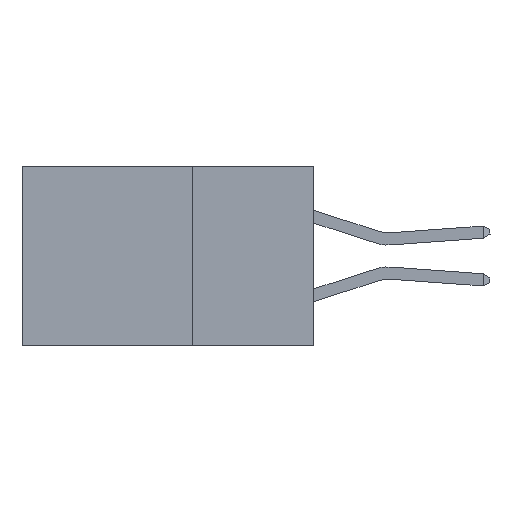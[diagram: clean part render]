
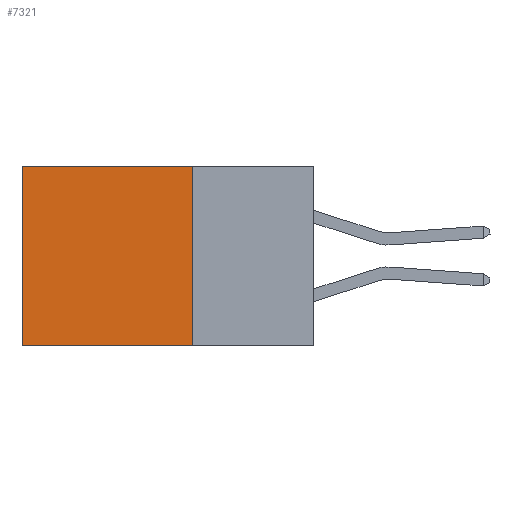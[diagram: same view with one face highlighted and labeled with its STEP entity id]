
A CAD part, left-side view. The second image highlights one B-rep face of the part: STEP entity #7321.
In plain terms, the highlighted planar face has unit normal (-1, 0, 0).
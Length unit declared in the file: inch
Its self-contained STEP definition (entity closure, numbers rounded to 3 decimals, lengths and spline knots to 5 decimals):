
#1502 = CARTESIAN_POINT ( 'NONE',  ( 0.2875, 0.6, -0.37 ) ) ;
#1985 = CARTESIAN_POINT ( 'NONE',  ( 0.2875, 0.6, 0. ) ) ;
#2287 = VECTOR ( 'NONE', #20335, 39.37008 ) ;
#2452 = PLANE ( 'NONE',  #14390 ) ;
#2771 = CARTESIAN_POINT ( 'NONE',  ( 0.2875, 0.25, -0.37 ) ) ;
#2923 = LINE ( 'NONE', #24197, #16357 ) ;
#5736 = DIRECTION ( 'NONE',  ( 0., 1., 0. ) ) ;
#6703 = CARTESIAN_POINT ( 'NONE',  ( 0.2875, 0.6, 0. ) ) ;
#6955 = EDGE_CURVE ( 'NONE', #21596, #11870, #9069, .T. ) ;
#7278 = CARTESIAN_POINT ( 'NONE',  ( 0.2875, 0.25, 0. ) ) ;
#7321 = ADVANCED_FACE ( 'NONE', ( #8411 ), #2452, .F. ) ;
#7917 = VERTEX_POINT ( 'NONE', #2771 ) ;
#8115 = VECTOR ( 'NONE', #5736, 39.37008 ) ;
#8411 = FACE_OUTER_BOUND ( 'NONE', #21296, .T. ) ;
#9069 = LINE ( 'NONE', #9857, #8115 ) ;
#9631 = VECTOR ( 'NONE', #17303, 39.37008 ) ;
#9857 = CARTESIAN_POINT ( 'NONE',  ( 0.2875, 0.25, 0. ) ) ;
#10536 = DIRECTION ( 'NONE',  ( 0., 0., -1. ) ) ;
#11357 = CARTESIAN_POINT ( 'NONE',  ( 0.2875, 0.25, 0. ) ) ;
#11870 = VERTEX_POINT ( 'NONE', #1985 ) ;
#13164 = ORIENTED_EDGE ( 'NONE', *, *, #19389, .F. ) ;
#13732 = EDGE_CURVE ( 'NONE', #7917, #23279, #2923, .T. ) ;
#13755 = EDGE_CURVE ( 'NONE', #11870, #23279, #14183, .T. ) ;
#14183 = LINE ( 'NONE', #6703, #2287 ) ;
#14256 = ORIENTED_EDGE ( 'NONE', *, *, #13755, .T. ) ;
#14390 = AXIS2_PLACEMENT_3D ( 'NONE', #22550, #16701, #10536 ) ;
#16116 = ORIENTED_EDGE ( 'NONE', *, *, #6955, .T. ) ;
#16165 = LINE ( 'NONE', #7278, #9631 ) ;
#16357 = VECTOR ( 'NONE', #18230, 39.37008 ) ;
#16701 = DIRECTION ( 'NONE',  ( 1., 0., 0. ) ) ;
#17303 = DIRECTION ( 'NONE',  ( 0., 0., -1. ) ) ;
#17551 = ORIENTED_EDGE ( 'NONE', *, *, #13732, .F. ) ;
#18230 = DIRECTION ( 'NONE',  ( 0., 1., 0. ) ) ;
#19389 = EDGE_CURVE ( 'NONE', #21596, #7917, #16165, .T. ) ;
#20335 = DIRECTION ( 'NONE',  ( 0., 0., -1. ) ) ;
#21296 = EDGE_LOOP ( 'NONE', ( #14256, #17551, #13164, #16116 ) ) ;
#21596 = VERTEX_POINT ( 'NONE', #11357 ) ;
#22550 = CARTESIAN_POINT ( 'NONE',  ( 0.2875, 0.25, 0. ) ) ;
#23279 = VERTEX_POINT ( 'NONE', #1502 ) ;
#24197 = CARTESIAN_POINT ( 'NONE',  ( 0.2875, 0.25, -0.37 ) ) ;
